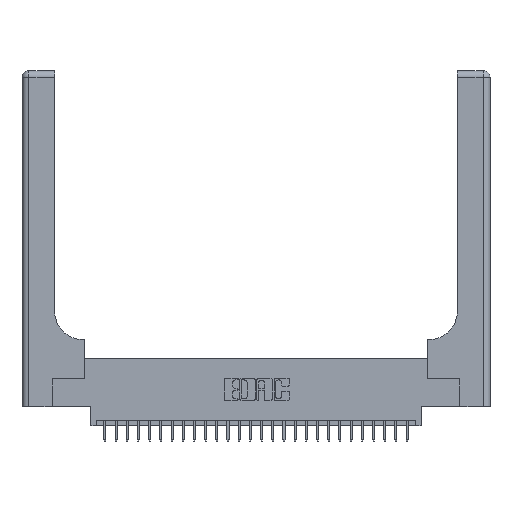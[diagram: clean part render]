
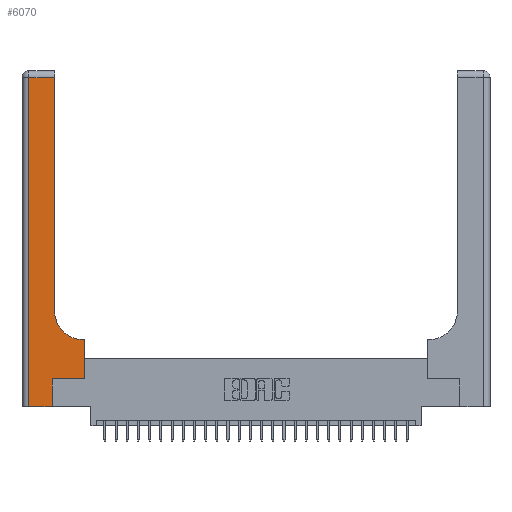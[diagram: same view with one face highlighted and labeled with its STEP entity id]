
A CAD part, top view. The second image highlights one B-rep face of the part: STEP entity #6070.
In plain terms, the highlighted planar face has unit normal (0, 0, 1).
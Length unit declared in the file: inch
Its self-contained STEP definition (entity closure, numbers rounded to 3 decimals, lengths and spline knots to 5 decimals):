
#828 = VECTOR ( 'NONE', #19532, 39.37008 ) ;
#1025 = EDGE_CURVE ( 'NONE', #12884, #24333, #28288, .T. ) ;
#1354 = CARTESIAN_POINT ( 'NONE',  ( 0.2915, 0.85, 0.37 ) ) ;
#1449 = VECTOR ( 'NONE', #26968, 39.37008 ) ;
#1662 = CARTESIAN_POINT ( 'NONE',  ( 0.2915, 2.94, 0.37 ) ) ;
#1740 = CARTESIAN_POINT ( 'NONE',  ( 0., 0., 0.37 ) ) ;
#2317 = VERTEX_POINT ( 'NONE', #6853 ) ;
#2449 = VERTEX_POINT ( 'NONE', #9377 ) ;
#3188 = CARTESIAN_POINT ( 'NONE',  ( 0.06, 3., 0.37 ) ) ;
#3344 = CIRCLE ( 'NONE', #17510, 0.25 ) ;
#3875 = DIRECTION ( 'NONE',  ( -1., 0., 0. ) ) ;
#5186 = EDGE_LOOP ( 'NONE', ( #16210, #21238, #11486, #8796, #21428, #17875, #14333, #16561, #7152 ) ) ;
#5391 = EDGE_CURVE ( 'NONE', #2449, #9299, #6511, .T. ) ;
#5434 = LINE ( 'NONE', #3188, #6450 ) ;
#5690 = DIRECTION ( 'NONE',  ( 1., 0., 0. ) ) ;
#5938 = VECTOR ( 'NONE', #9636, 39.37008 ) ;
#6070 = ADVANCED_FACE ( 'NONE', ( #15289 ), #13367, .F. ) ;
#6450 = VECTOR ( 'NONE', #12262, 39.37008 ) ;
#6511 = LINE ( 'NONE', #24962, #9314 ) ;
#6853 = CARTESIAN_POINT ( 'NONE',  ( 0.06, 0., 0.37 ) ) ;
#7152 = ORIENTED_EDGE ( 'NONE', *, *, #10708, .T. ) ;
#7514 = EDGE_CURVE ( 'NONE', #15945, #12884, #19100, .T. ) ;
#7998 = CARTESIAN_POINT ( 'NONE',  ( 0.06, 2.94, 0.37 ) ) ;
#8647 = DIRECTION ( 'NONE',  ( -1., 0., 0. ) ) ;
#8796 = ORIENTED_EDGE ( 'NONE', *, *, #8897, .T. ) ;
#8897 = EDGE_CURVE ( 'NONE', #2317, #2449, #14950, .T. ) ;
#9299 = VERTEX_POINT ( 'NONE', #27132 ) ;
#9314 = VECTOR ( 'NONE', #20658, 39.37008 ) ;
#9377 = CARTESIAN_POINT ( 'NONE',  ( 0.269, 0., 0.37 ) ) ;
#9636 = DIRECTION ( 'NONE',  ( 1., 0., 0. ) ) ;
#10132 = LINE ( 'NONE', #19094, #24659 ) ;
#10708 = EDGE_CURVE ( 'NONE', #24333, #13377, #3344, .T. ) ;
#11136 = CARTESIAN_POINT ( 'NONE',  ( 0., 3., 0.37 ) ) ;
#11486 = ORIENTED_EDGE ( 'NONE', *, *, #25846, .T. ) ;
#11697 = AXIS2_PLACEMENT_3D ( 'NONE', #11136, #28867, #8647 ) ;
#11856 = LINE ( 'NONE', #19296, #5938 ) ;
#12007 = CARTESIAN_POINT ( 'NONE',  ( 0.5415, 0.6, 0.37 ) ) ;
#12262 = DIRECTION ( 'NONE',  ( 0., -1., 0. ) ) ;
#12884 = VERTEX_POINT ( 'NONE', #26871 ) ;
#13036 = DIRECTION ( 'NONE',  ( 1., 0., 0. ) ) ;
#13367 = PLANE ( 'NONE',  #11697 ) ;
#13377 = VERTEX_POINT ( 'NONE', #1354 ) ;
#13544 = CARTESIAN_POINT ( 'NONE',  ( 0., 2.94, 0.37 ) ) ;
#14333 = ORIENTED_EDGE ( 'NONE', *, *, #7514, .T. ) ;
#14873 = VECTOR ( 'NONE', #3875, 39.37008 ) ;
#14950 = LINE ( 'NONE', #1740, #21195 ) ;
#15148 = CARTESIAN_POINT ( 'NONE',  ( 0.5585, 0.25, 0.37 ) ) ;
#15289 = FACE_OUTER_BOUND ( 'NONE', #5186, .T. ) ;
#15515 = EDGE_CURVE ( 'NONE', #17652, #22270, #29054, .T. ) ;
#15945 = VERTEX_POINT ( 'NONE', #15148 ) ;
#16210 = ORIENTED_EDGE ( 'NONE', *, *, #19120, .T. ) ;
#16561 = ORIENTED_EDGE ( 'NONE', *, *, #1025, .T. ) ;
#17188 = DIRECTION ( 'NONE',  ( 0., 0., -1. ) ) ;
#17510 = AXIS2_PLACEMENT_3D ( 'NONE', #25942, #17188, #5690 ) ;
#17652 = VERTEX_POINT ( 'NONE', #1662 ) ;
#17875 = ORIENTED_EDGE ( 'NONE', *, *, #23117, .T. ) ;
#19094 = CARTESIAN_POINT ( 'NONE',  ( 0.2915, 3., 0.37 ) ) ;
#19100 = LINE ( 'NONE', #19394, #828 ) ;
#19120 = EDGE_CURVE ( 'NONE', #13377, #17652, #10132, .T. ) ;
#19296 = CARTESIAN_POINT ( 'NONE',  ( 0.269, 0.25, 0.37 ) ) ;
#19394 = CARTESIAN_POINT ( 'NONE',  ( 0.5585, 0.25, 0.37 ) ) ;
#19532 = DIRECTION ( 'NONE',  ( 0., 1., 0. ) ) ;
#20658 = DIRECTION ( 'NONE',  ( 0., 1., 0. ) ) ;
#21195 = VECTOR ( 'NONE', #13036, 39.37008 ) ;
#21238 = ORIENTED_EDGE ( 'NONE', *, *, #15515, .T. ) ;
#21428 = ORIENTED_EDGE ( 'NONE', *, *, #5391, .T. ) ;
#22270 = VERTEX_POINT ( 'NONE', #7998 ) ;
#23117 = EDGE_CURVE ( 'NONE', #9299, #15945, #11856, .T. ) ;
#24333 = VERTEX_POINT ( 'NONE', #12007 ) ;
#24659 = VECTOR ( 'NONE', #28133, 39.37008 ) ;
#24962 = CARTESIAN_POINT ( 'NONE',  ( 0.269, 0., 0.37 ) ) ;
#25846 = EDGE_CURVE ( 'NONE', #22270, #2317, #5434, .T. ) ;
#25942 = CARTESIAN_POINT ( 'NONE',  ( 0.5415, 0.85, 0.37 ) ) ;
#25947 = CARTESIAN_POINT ( 'NONE',  ( 0.2915, 0.6, 0.37 ) ) ;
#26871 = CARTESIAN_POINT ( 'NONE',  ( 0.5585, 0.6, 0.37 ) ) ;
#26968 = DIRECTION ( 'NONE',  ( -1., 0., 0. ) ) ;
#27132 = CARTESIAN_POINT ( 'NONE',  ( 0.269, 0.25, 0.37 ) ) ;
#28133 = DIRECTION ( 'NONE',  ( 0., 1., 0. ) ) ;
#28288 = LINE ( 'NONE', #25947, #14873 ) ;
#28867 = DIRECTION ( 'NONE',  ( 0., 0., -1. ) ) ;
#29054 = LINE ( 'NONE', #13544, #1449 ) ;
